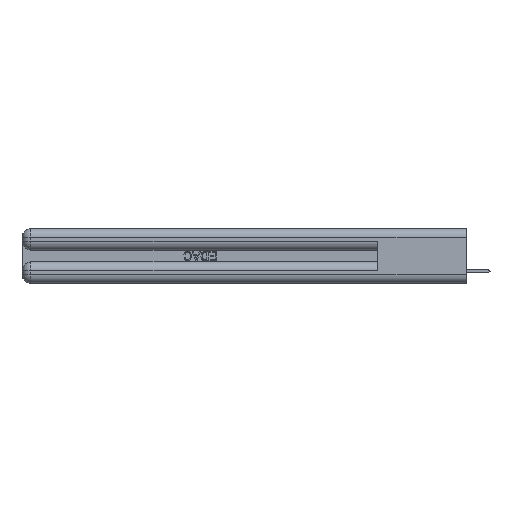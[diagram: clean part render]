
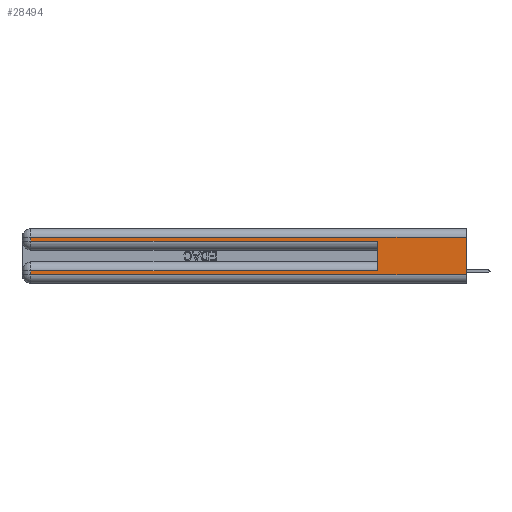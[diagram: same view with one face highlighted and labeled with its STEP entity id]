
A CAD part, left-side view. The second image highlights one B-rep face of the part: STEP entity #28494.
In plain terms, the highlighted planar face has unit normal (-1, 0, 0).
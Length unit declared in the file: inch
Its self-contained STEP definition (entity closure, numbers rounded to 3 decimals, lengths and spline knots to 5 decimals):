
#55 = EDGE_LOOP ( 'NONE', ( #7196, #34109, #8691, #34030, #20220, #27741, #23452, #2875 ) ) ;
#509 = VECTOR ( 'NONE', #29226, 39.37008 ) ;
#649 = CARTESIAN_POINT ( 'NONE',  ( 0., 2.94, 0.085 ) ) ;
#1321 = CARTESIAN_POINT ( 'NONE',  ( 0., 2.94, 0.37 ) ) ;
#1880 = LINE ( 'NONE', #19806, #33462 ) ;
#2875 = ORIENTED_EDGE ( 'NONE', *, *, #40173, .T. ) ;
#2961 = EDGE_CURVE ( 'NONE', #18232, #27913, #1880, .T. ) ;
#3021 = LINE ( 'NONE', #9246, #20644 ) ;
#3235 = EDGE_CURVE ( 'NONE', #22980, #16752, #13583, .T. ) ;
#3487 = LINE ( 'NONE', #13078, #10986 ) ;
#5562 = VECTOR ( 'NONE', #44088, 39.37008 ) ;
#7196 = ORIENTED_EDGE ( 'NONE', *, *, #31964, .F. ) ;
#8462 = CARTESIAN_POINT ( 'NONE',  ( 0., 0., 0.31 ) ) ;
#8691 = ORIENTED_EDGE ( 'NONE', *, *, #40018, .T. ) ;
#9246 = CARTESIAN_POINT ( 'NONE',  ( 0., 0., 0.06 ) ) ;
#10789 = VERTEX_POINT ( 'NONE', #12830 ) ;
#10986 = VECTOR ( 'NONE', #40439, 39.37008 ) ;
#11928 = CARTESIAN_POINT ( 'NONE',  ( 0., 2.94, 0.31 ) ) ;
#12096 = LINE ( 'NONE', #41427, #28173 ) ;
#12830 = CARTESIAN_POINT ( 'NONE',  ( 0., 2.94, 0.285 ) ) ;
#13078 = CARTESIAN_POINT ( 'NONE',  ( 0., 0., 0.37 ) ) ;
#13583 = LINE ( 'NONE', #8462, #5562 ) ;
#14982 = LINE ( 'NONE', #15692, #509 ) ;
#15663 = DIRECTION ( 'NONE',  ( 0., -1., 0. ) ) ;
#15692 = CARTESIAN_POINT ( 'NONE',  ( 0., 0., 0.285 ) ) ;
#16752 = VERTEX_POINT ( 'NONE', #11928 ) ;
#18232 = VERTEX_POINT ( 'NONE', #649 ) ;
#19806 = CARTESIAN_POINT ( 'NONE',  ( 0., 2.94, 0.37 ) ) ;
#20220 = ORIENTED_EDGE ( 'NONE', *, *, #28404, .F. ) ;
#20644 = VECTOR ( 'NONE', #15663, 39.37008 ) ;
#21566 = PLANE ( 'NONE',  #27329 ) ;
#22487 = DIRECTION ( 'NONE',  ( 0., 0., -1. ) ) ;
#22980 = VERTEX_POINT ( 'NONE', #44098 ) ;
#23392 = LINE ( 'NONE', #1321, #40974 ) ;
#23452 = ORIENTED_EDGE ( 'NONE', *, *, #2961, .T. ) ;
#24795 = VECTOR ( 'NONE', #39537, 39.37008 ) ;
#25573 = DIRECTION ( 'NONE',  ( 0., 0., -1. ) ) ;
#25840 = CARTESIAN_POINT ( 'NONE',  ( 0., 0.6, 0.145 ) ) ;
#27329 = AXIS2_PLACEMENT_3D ( 'NONE', #31853, #28760, #22487 ) ;
#27341 = CARTESIAN_POINT ( 'NONE',  ( 0., 0.6, 0.285 ) ) ;
#27741 = ORIENTED_EDGE ( 'NONE', *, *, #41185, .T. ) ;
#27902 = VERTEX_POINT ( 'NONE', #41819 ) ;
#27913 = VERTEX_POINT ( 'NONE', #41513 ) ;
#28023 = DIRECTION ( 'NONE',  ( 0., 1., 0. ) ) ;
#28173 = VECTOR ( 'NONE', #28023, 39.37008 ) ;
#28404 = EDGE_CURVE ( 'NONE', #27902, #35998, #33917, .T. ) ;
#28494 = ADVANCED_FACE ( 'NONE', ( #42489 ), #21566, .F. ) ;
#28760 = DIRECTION ( 'NONE',  ( 1., 0., 0. ) ) ;
#29226 = DIRECTION ( 'NONE',  ( 0., -1., 0. ) ) ;
#31853 = CARTESIAN_POINT ( 'NONE',  ( 0., 0., 0.37 ) ) ;
#31964 = EDGE_CURVE ( 'NONE', #22980, #43137, #3487, .T. ) ;
#33462 = VECTOR ( 'NONE', #33537, 39.37008 ) ;
#33537 = DIRECTION ( 'NONE',  ( 0., 0., -1. ) ) ;
#33917 = LINE ( 'NONE', #25840, #24795 ) ;
#34030 = ORIENTED_EDGE ( 'NONE', *, *, #38079, .T. ) ;
#34109 = ORIENTED_EDGE ( 'NONE', *, *, #3235, .T. ) ;
#35998 = VERTEX_POINT ( 'NONE', #27341 ) ;
#38079 = EDGE_CURVE ( 'NONE', #10789, #35998, #14982, .T. ) ;
#39279 = CARTESIAN_POINT ( 'NONE',  ( 0., 0., 0.06 ) ) ;
#39537 = DIRECTION ( 'NONE',  ( 0., 0., 1. ) ) ;
#40018 = EDGE_CURVE ( 'NONE', #16752, #10789, #23392, .T. ) ;
#40173 = EDGE_CURVE ( 'NONE', #27913, #43137, #3021, .T. ) ;
#40439 = DIRECTION ( 'NONE',  ( 0., 0., -1. ) ) ;
#40974 = VECTOR ( 'NONE', #25573, 39.37008 ) ;
#41185 = EDGE_CURVE ( 'NONE', #27902, #18232, #12096, .T. ) ;
#41427 = CARTESIAN_POINT ( 'NONE',  ( 0., 0., 0.085 ) ) ;
#41513 = CARTESIAN_POINT ( 'NONE',  ( 0., 2.94, 0.06 ) ) ;
#41819 = CARTESIAN_POINT ( 'NONE',  ( 0., 0.6, 0.085 ) ) ;
#42489 = FACE_OUTER_BOUND ( 'NONE', #55, .T. ) ;
#43137 = VERTEX_POINT ( 'NONE', #39279 ) ;
#44088 = DIRECTION ( 'NONE',  ( 0., 1., 0. ) ) ;
#44098 = CARTESIAN_POINT ( 'NONE',  ( 0., 0., 0.31 ) ) ;
